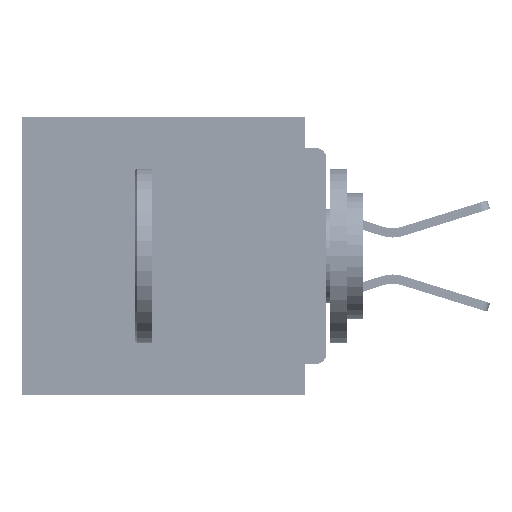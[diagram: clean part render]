
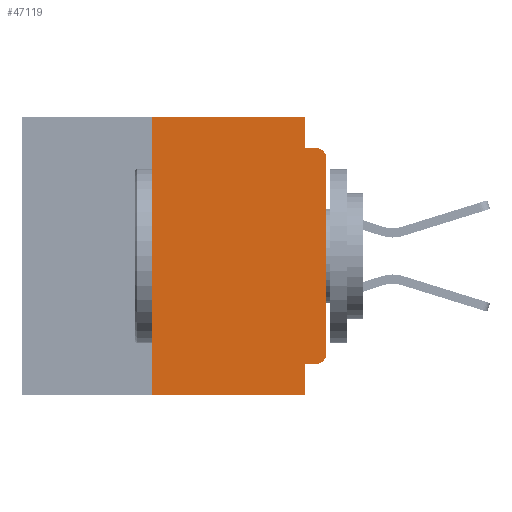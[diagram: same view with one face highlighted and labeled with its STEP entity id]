
A CAD part, left-side view. The second image highlights one B-rep face of the part: STEP entity #47119.
In plain terms, the highlighted planar face has unit normal (-1, 0, 0).
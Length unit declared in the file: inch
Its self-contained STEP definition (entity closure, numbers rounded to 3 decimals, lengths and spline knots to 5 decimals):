
#198 = ORIENTED_EDGE ( 'NONE', *, *, #63893, .F. ) ;
#1022 = CARTESIAN_POINT ( 'NONE',  ( 0., 0., -0.045 ) ) ;
#1323 = LINE ( 'NONE', #66084, #55744 ) ;
#3561 = DIRECTION ( 'NONE',  ( 0., 0., -1. ) ) ;
#3745 = CARTESIAN_POINT ( 'NONE',  ( 0., 0.015, -0.355 ) ) ;
#3965 = AXIS2_PLACEMENT_3D ( 'NONE', #66562, #35209, #3561 ) ;
#4022 = DIRECTION ( 'NONE',  ( 0., 0., -1. ) ) ;
#4108 = EDGE_LOOP ( 'NONE', ( #10655, #20634, #60881, #49525, #66869, #198, #9926, #55562, #63480, #4495 ) ) ;
#4428 = VERTEX_POINT ( 'NONE', #58687 ) ;
#4495 = ORIENTED_EDGE ( 'NONE', *, *, #48113, .T. ) ;
#4591 = DIRECTION ( 'NONE',  ( 1., 0., 0. ) ) ;
#4641 = CARTESIAN_POINT ( 'NONE',  ( 0., 0.031, -0.045 ) ) ;
#6442 = LINE ( 'NONE', #25605, #18872 ) ;
#7494 = AXIS2_PLACEMENT_3D ( 'NONE', #14018, #50927, #19367 ) ;
#7728 = CIRCLE ( 'NONE', #7494, 0.015 ) ;
#9091 = LINE ( 'NONE', #1022, #61795 ) ;
#9406 = CARTESIAN_POINT ( 'NONE',  ( 0., 0., -0.34 ) ) ;
#9926 = ORIENTED_EDGE ( 'NONE', *, *, #51497, .T. ) ;
#10528 = CARTESIAN_POINT ( 'NONE',  ( 0., 0.437, -0.4 ) ) ;
#10655 = ORIENTED_EDGE ( 'NONE', *, *, #29788, .T. ) ;
#13731 = LINE ( 'NONE', #47472, #40234 ) ;
#14018 = CARTESIAN_POINT ( 'NONE',  ( 0., 0.015, -0.06 ) ) ;
#14265 = EDGE_CURVE ( 'NONE', #42446, #42863, #25065, .T. ) ;
#16371 = CARTESIAN_POINT ( 'NONE',  ( 0., 0.015, -0.045 ) ) ;
#17076 = DIRECTION ( 'NONE',  ( 0., 1., 0. ) ) ;
#17206 = VERTEX_POINT ( 'NONE', #4641 ) ;
#17842 = EDGE_CURVE ( 'NONE', #4428, #37055, #6442, .T. ) ;
#18872 = VECTOR ( 'NONE', #67557, 39.37008 ) ;
#19367 = DIRECTION ( 'NONE',  ( 0., 0., -1. ) ) ;
#19849 = AXIS2_PLACEMENT_3D ( 'NONE', #67585, #4591, #41574 ) ;
#20634 = ORIENTED_EDGE ( 'NONE', *, *, #31355, .T. ) ;
#22485 = VECTOR ( 'NONE', #50164, 39.37008 ) ;
#23695 = EDGE_CURVE ( 'NONE', #37055, #17206, #1323, .T. ) ;
#24643 = VERTEX_POINT ( 'NONE', #48905 ) ;
#25065 = LINE ( 'NONE', #53888, #53032 ) ;
#25605 = CARTESIAN_POINT ( 'NONE',  ( 0., 0.437, 0. ) ) ;
#25792 = LINE ( 'NONE', #44943, #22485 ) ;
#29788 = EDGE_CURVE ( 'NONE', #41352, #51026, #13731, .T. ) ;
#30931 = PLANE ( 'NONE',  #19849 ) ;
#31355 = EDGE_CURVE ( 'NONE', #51026, #50923, #7728, .T. ) ;
#31573 = DIRECTION ( 'NONE',  ( 0., -1., 0. ) ) ;
#32789 = DIRECTION ( 'NONE',  ( 0., 0., -1. ) ) ;
#35050 = CIRCLE ( 'NONE', #3965, 0.015 ) ;
#35209 = DIRECTION ( 'NONE',  ( -1., 0., 0. ) ) ;
#35277 = CARTESIAN_POINT ( 'NONE',  ( 0., 0.031, -0.4 ) ) ;
#36361 = VECTOR ( 'NONE', #32789, 39.37008 ) ;
#36676 = EDGE_CURVE ( 'NONE', #17206, #50923, #9091, .T. ) ;
#37055 = VERTEX_POINT ( 'NONE', #46035 ) ;
#40234 = VECTOR ( 'NONE', #52694, 39.37008 ) ;
#41352 = VERTEX_POINT ( 'NONE', #9406 ) ;
#41574 = DIRECTION ( 'NONE',  ( 0., 0., -1. ) ) ;
#41823 = FACE_OUTER_BOUND ( 'NONE', #4108, .T. ) ;
#42446 = VERTEX_POINT ( 'NONE', #3745 ) ;
#42851 = LINE ( 'NONE', #10528, #44499 ) ;
#42863 = VERTEX_POINT ( 'NONE', #43928 ) ;
#43928 = CARTESIAN_POINT ( 'NONE',  ( 0., 0.031, -0.355 ) ) ;
#44499 = VECTOR ( 'NONE', #31573, 39.37008 ) ;
#44943 = CARTESIAN_POINT ( 'NONE',  ( 0., 0.25, -0.4 ) ) ;
#46035 = CARTESIAN_POINT ( 'NONE',  ( 0., 0.031, 0. ) ) ;
#47119 = ADVANCED_FACE ( 'NONE', ( #41823 ), #30931, .F. ) ;
#47472 = CARTESIAN_POINT ( 'NONE',  ( 0., 0., 0. ) ) ;
#48113 = EDGE_CURVE ( 'NONE', #42446, #41352, #35050, .T. ) ;
#48905 = CARTESIAN_POINT ( 'NONE',  ( 0., 0.25, -0.4 ) ) ;
#49525 = ORIENTED_EDGE ( 'NONE', *, *, #23695, .F. ) ;
#50164 = DIRECTION ( 'NONE',  ( 0., 0., 1. ) ) ;
#50923 = VERTEX_POINT ( 'NONE', #16371 ) ;
#50927 = DIRECTION ( 'NONE',  ( -1., 0., 0. ) ) ;
#51026 = VERTEX_POINT ( 'NONE', #53646 ) ;
#51497 = EDGE_CURVE ( 'NONE', #24643, #62559, #42851, .T. ) ;
#52694 = DIRECTION ( 'NONE',  ( 0., 0., 1. ) ) ;
#53032 = VECTOR ( 'NONE', #17076, 39.37008 ) ;
#53646 = CARTESIAN_POINT ( 'NONE',  ( 0., 0., -0.06 ) ) ;
#53888 = CARTESIAN_POINT ( 'NONE',  ( 0., 0., -0.355 ) ) ;
#53895 = CARTESIAN_POINT ( 'NONE',  ( 0., 0.031, -0.4 ) ) ;
#55562 = ORIENTED_EDGE ( 'NONE', *, *, #67882, .F. ) ;
#55744 = VECTOR ( 'NONE', #4022, 39.37008 ) ;
#58687 = CARTESIAN_POINT ( 'NONE',  ( 0., 0.25, 0. ) ) ;
#59053 = DIRECTION ( 'NONE',  ( 0., -1., 0. ) ) ;
#60881 = ORIENTED_EDGE ( 'NONE', *, *, #36676, .F. ) ;
#61795 = VECTOR ( 'NONE', #59053, 39.37008 ) ;
#62559 = VERTEX_POINT ( 'NONE', #35277 ) ;
#63480 = ORIENTED_EDGE ( 'NONE', *, *, #14265, .F. ) ;
#63893 = EDGE_CURVE ( 'NONE', #24643, #4428, #25792, .T. ) ;
#64216 = LINE ( 'NONE', #53895, #36361 ) ;
#66084 = CARTESIAN_POINT ( 'NONE',  ( 0., 0.031, 0. ) ) ;
#66562 = CARTESIAN_POINT ( 'NONE',  ( 0., 0.015, -0.34 ) ) ;
#66869 = ORIENTED_EDGE ( 'NONE', *, *, #17842, .F. ) ;
#67557 = DIRECTION ( 'NONE',  ( 0., -1., 0. ) ) ;
#67585 = CARTESIAN_POINT ( 'NONE',  ( 0., 0.437, 0. ) ) ;
#67882 = EDGE_CURVE ( 'NONE', #42863, #62559, #64216, .T. ) ;
